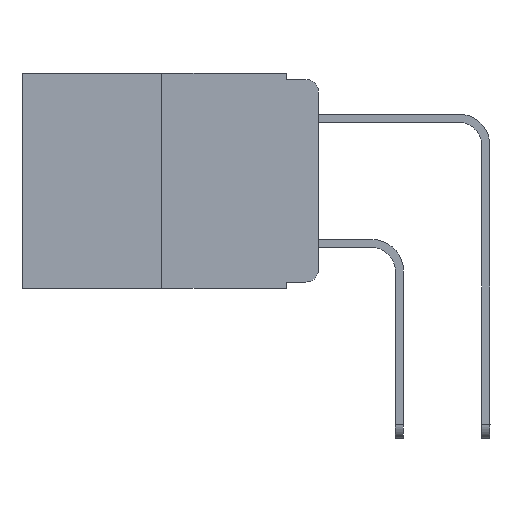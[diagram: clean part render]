
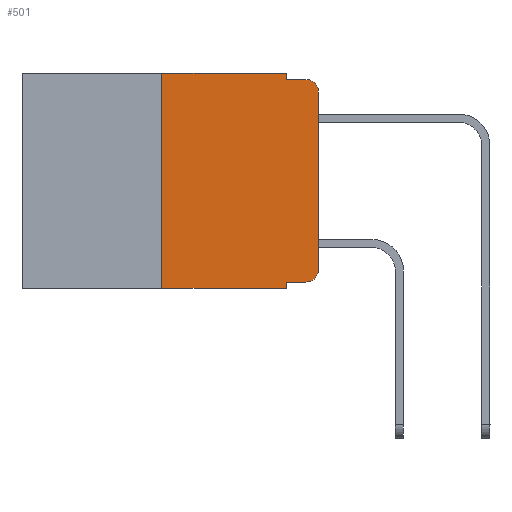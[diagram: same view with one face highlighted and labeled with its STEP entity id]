
A CAD part, left-side view. The second image highlights one B-rep face of the part: STEP entity #501.
In plain terms, the highlighted planar face has unit normal (-1, 0, 0).
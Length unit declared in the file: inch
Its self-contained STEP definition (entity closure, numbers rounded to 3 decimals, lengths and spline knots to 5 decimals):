
#77 = CARTESIAN_POINT ( 'NONE',  ( 0., 0.051, -0.333 ) ) ;
#315 = LINE ( 'NONE', #13027, #11624 ) ;
#491 = CARTESIAN_POINT ( 'NONE',  ( 0., 0.051, 0. ) ) ;
#501 = ADVANCED_FACE ( 'NONE', ( #11183 ), #2814, .F. ) ;
#777 = VERTEX_POINT ( 'NONE', #8409 ) ;
#1004 = DIRECTION ( 'NONE',  ( 0., -1., 0. ) ) ;
#1344 = CARTESIAN_POINT ( 'NONE',  ( 0., 0.25, 0. ) ) ;
#1465 = EDGE_CURVE ( 'NONE', #5921, #5255, #2217, .T. ) ;
#1877 = AXIS2_PLACEMENT_3D ( 'NONE', #5375, #8449, #7455 ) ;
#2066 = EDGE_CURVE ( 'NONE', #7864, #11693, #5842, .T. ) ;
#2217 = LINE ( 'NONE', #4419, #13169 ) ;
#2258 = CARTESIAN_POINT ( 'NONE',  ( 0., 0.02, -0.01 ) ) ;
#2272 = CARTESIAN_POINT ( 'NONE',  ( 0., 0.051, 0. ) ) ;
#2378 = AXIS2_PLACEMENT_3D ( 'NONE', #6074, #7288, #3559 ) ;
#2632 = EDGE_CURVE ( 'NONE', #12407, #777, #13585, .T. ) ;
#2814 = PLANE ( 'NONE',  #1877 ) ;
#2871 = EDGE_CURVE ( 'NONE', #11693, #6143, #8538, .T. ) ;
#3172 = EDGE_CURVE ( 'NONE', #7864, #8151, #12730, .T. ) ;
#3345 = CIRCLE ( 'NONE', #2378, 0.02 ) ;
#3430 = VECTOR ( 'NONE', #8846, 39.37008 ) ;
#3552 = LINE ( 'NONE', #2272, #14580 ) ;
#3559 = DIRECTION ( 'NONE',  ( 0., 0., -1. ) ) ;
#3625 = CARTESIAN_POINT ( 'NONE',  ( 0., 0.25, 0. ) ) ;
#4026 = ORIENTED_EDGE ( 'NONE', *, *, #2632, .T. ) ;
#4180 = ORIENTED_EDGE ( 'NONE', *, *, #8552, .F. ) ;
#4197 = VECTOR ( 'NONE', #6903, 39.37008 ) ;
#4419 = CARTESIAN_POINT ( 'NONE',  ( 0., 0.051, -0.01 ) ) ;
#5198 = ORIENTED_EDGE ( 'NONE', *, *, #11156, .T. ) ;
#5255 = VERTEX_POINT ( 'NONE', #2258 ) ;
#5375 = CARTESIAN_POINT ( 'NONE',  ( 0., 0.473, 0. ) ) ;
#5684 = ORIENTED_EDGE ( 'NONE', *, *, #3172, .T. ) ;
#5770 = CARTESIAN_POINT ( 'NONE',  ( 0., 0.473, -0.343 ) ) ;
#5842 = LINE ( 'NONE', #3625, #12673 ) ;
#5917 = DIRECTION ( 'NONE',  ( 0., 0., -1. ) ) ;
#5921 = VERTEX_POINT ( 'NONE', #9694 ) ;
#5932 = CARTESIAN_POINT ( 'NONE',  ( 0., 0.473, 0. ) ) ;
#6074 = CARTESIAN_POINT ( 'NONE',  ( 0., 0.02, -0.313 ) ) ;
#6143 = VERTEX_POINT ( 'NONE', #12873 ) ;
#6540 = VERTEX_POINT ( 'NONE', #77 ) ;
#6586 = VECTOR ( 'NONE', #10755, 39.37008 ) ;
#6676 = CARTESIAN_POINT ( 'NONE',  ( 0., 0.02, -0.333 ) ) ;
#6903 = DIRECTION ( 'NONE',  ( 0., -1., 0. ) ) ;
#7229 = CARTESIAN_POINT ( 'NONE',  ( 0., 0.02, -0.03 ) ) ;
#7288 = DIRECTION ( 'NONE',  ( -1., 0., 0. ) ) ;
#7377 = ORIENTED_EDGE ( 'NONE', *, *, #2871, .F. ) ;
#7397 = DIRECTION ( 'NONE',  ( -1., 0., 0. ) ) ;
#7455 = DIRECTION ( 'NONE',  ( 0., 0., -1. ) ) ;
#7511 = EDGE_CURVE ( 'NONE', #777, #5255, #10216, .T. ) ;
#7864 = VERTEX_POINT ( 'NONE', #11151 ) ;
#8151 = VERTEX_POINT ( 'NONE', #10595 ) ;
#8289 = ORIENTED_EDGE ( 'NONE', *, *, #10880, .F. ) ;
#8409 = CARTESIAN_POINT ( 'NONE',  ( 0., 0., -0.03 ) ) ;
#8449 = DIRECTION ( 'NONE',  ( 1., 0., 0. ) ) ;
#8538 = LINE ( 'NONE', #5932, #6586 ) ;
#8552 = EDGE_CURVE ( 'NONE', #6143, #5921, #3552, .T. ) ;
#8846 = DIRECTION ( 'NONE',  ( 0., 0., 1. ) ) ;
#9175 = VECTOR ( 'NONE', #13571, 39.37008 ) ;
#9427 = DIRECTION ( 'NONE',  ( 0., 0., 1. ) ) ;
#9694 = CARTESIAN_POINT ( 'NONE',  ( 0., 0.051, -0.01 ) ) ;
#10216 = CIRCLE ( 'NONE', #12170, 0.02 ) ;
#10595 = CARTESIAN_POINT ( 'NONE',  ( 0., 0.051, -0.343 ) ) ;
#10606 = CARTESIAN_POINT ( 'NONE',  ( 0., 0., -0.313 ) ) ;
#10755 = DIRECTION ( 'NONE',  ( 0., -1., 0. ) ) ;
#10880 = EDGE_CURVE ( 'NONE', #6540, #8151, #12217, .T. ) ;
#11087 = CARTESIAN_POINT ( 'NONE',  ( 0., 0., 0. ) ) ;
#11151 = CARTESIAN_POINT ( 'NONE',  ( 0., 0.25, -0.343 ) ) ;
#11156 = EDGE_CURVE ( 'NONE', #14271, #12407, #3345, .T. ) ;
#11183 = FACE_OUTER_BOUND ( 'NONE', #11379, .T. ) ;
#11199 = EDGE_CURVE ( 'NONE', #6540, #14271, #315, .T. ) ;
#11379 = EDGE_LOOP ( 'NONE', ( #4026, #12121, #14875, #4180, #7377, #12777, #5684, #8289, #12988, #5198 ) ) ;
#11624 = VECTOR ( 'NONE', #11961, 39.37008 ) ;
#11693 = VERTEX_POINT ( 'NONE', #1344 ) ;
#11816 = DIRECTION ( 'NONE',  ( 0., 0., -1. ) ) ;
#11961 = DIRECTION ( 'NONE',  ( 0., -1., 0. ) ) ;
#12121 = ORIENTED_EDGE ( 'NONE', *, *, #7511, .T. ) ;
#12170 = AXIS2_PLACEMENT_3D ( 'NONE', #7229, #7397, #11816 ) ;
#12217 = LINE ( 'NONE', #491, #9175 ) ;
#12407 = VERTEX_POINT ( 'NONE', #10606 ) ;
#12673 = VECTOR ( 'NONE', #9427, 39.37008 ) ;
#12730 = LINE ( 'NONE', #5770, #4197 ) ;
#12777 = ORIENTED_EDGE ( 'NONE', *, *, #2066, .F. ) ;
#12873 = CARTESIAN_POINT ( 'NONE',  ( 0., 0.051, 0. ) ) ;
#12988 = ORIENTED_EDGE ( 'NONE', *, *, #11199, .T. ) ;
#13027 = CARTESIAN_POINT ( 'NONE',  ( 0., 0.051, -0.333 ) ) ;
#13169 = VECTOR ( 'NONE', #1004, 39.37008 ) ;
#13571 = DIRECTION ( 'NONE',  ( 0., 0., -1. ) ) ;
#13585 = LINE ( 'NONE', #11087, #3430 ) ;
#14271 = VERTEX_POINT ( 'NONE', #6676 ) ;
#14580 = VECTOR ( 'NONE', #5917, 39.37008 ) ;
#14875 = ORIENTED_EDGE ( 'NONE', *, *, #1465, .F. ) ;
